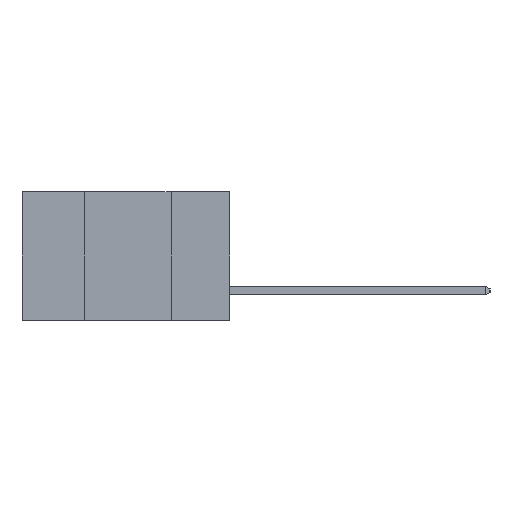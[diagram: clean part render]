
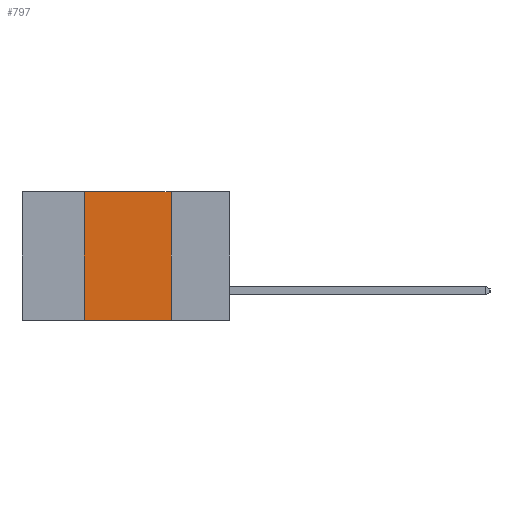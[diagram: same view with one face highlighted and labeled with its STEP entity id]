
A CAD part, left-side view. The second image highlights one B-rep face of the part: STEP entity #797.
In plain terms, the highlighted planar face has unit normal (-1, 0, 0).
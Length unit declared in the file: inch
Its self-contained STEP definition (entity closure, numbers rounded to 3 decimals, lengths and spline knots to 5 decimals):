
#316 = DIRECTION ( 'NONE',  ( 0., -1., 0. ) ) ;
#605 = DIRECTION ( 'NONE',  ( 0., 0., -1. ) ) ;
#797 = ADVANCED_FACE ( 'NONE', ( #4224 ), #5709, .F. ) ;
#1355 = DIRECTION ( 'NONE',  ( 0., 0., -1. ) ) ;
#2136 = DIRECTION ( 'NONE',  ( 1., 0., 0. ) ) ;
#2278 = CARTESIAN_POINT ( 'NONE',  ( 0., 0.17, 0. ) ) ;
#2495 = VERTEX_POINT ( 'NONE', #7505 ) ;
#2647 = AXIS2_PLACEMENT_3D ( 'NONE', #14229, #2136, #1355 ) ;
#2806 = EDGE_CURVE ( 'NONE', #2495, #14706, #14715, .T. ) ;
#3045 = VECTOR ( 'NONE', #605, 39.37008 ) ;
#4089 = ORIENTED_EDGE ( 'NONE', *, *, #2806, .F. ) ;
#4102 = CARTESIAN_POINT ( 'NONE',  ( 0., 0.17, -0.37 ) ) ;
#4224 = FACE_OUTER_BOUND ( 'NONE', #4238, .T. ) ;
#4238 = EDGE_LOOP ( 'NONE', ( #6696, #4089, #9150, #4244 ) ) ;
#4244 = ORIENTED_EDGE ( 'NONE', *, *, #5163, .T. ) ;
#4449 = CARTESIAN_POINT ( 'NONE',  ( 0., 0.42, -0.37 ) ) ;
#4867 = CARTESIAN_POINT ( 'NONE',  ( 0., 0.42, 0. ) ) ;
#5163 = EDGE_CURVE ( 'NONE', #10634, #12291, #5690, .T. ) ;
#5690 = LINE ( 'NONE', #10066, #6448 ) ;
#5709 = PLANE ( 'NONE',  #2647 ) ;
#6445 = DIRECTION ( 'NONE',  ( 0., -1., 0. ) ) ;
#6448 = VECTOR ( 'NONE', #6445, 39.37008 ) ;
#6559 = CARTESIAN_POINT ( 'NONE',  ( 0., 0.17, 0. ) ) ;
#6696 = ORIENTED_EDGE ( 'NONE', *, *, #11804, .F. ) ;
#7505 = CARTESIAN_POINT ( 'NONE',  ( 0., 0.42, 0. ) ) ;
#9150 = ORIENTED_EDGE ( 'NONE', *, *, #12096, .F. ) ;
#10066 = CARTESIAN_POINT ( 'NONE',  ( 0., 0.6, -0.37 ) ) ;
#10634 = VERTEX_POINT ( 'NONE', #4449 ) ;
#10825 = DIRECTION ( 'NONE',  ( 0., 0., 1. ) ) ;
#11586 = VECTOR ( 'NONE', #316, 39.37008 ) ;
#11804 = EDGE_CURVE ( 'NONE', #14706, #12291, #12485, .T. ) ;
#12096 = EDGE_CURVE ( 'NONE', #10634, #2495, #14315, .T. ) ;
#12291 = VERTEX_POINT ( 'NONE', #4102 ) ;
#12445 = CARTESIAN_POINT ( 'NONE',  ( 0., 0.6, 0. ) ) ;
#12485 = LINE ( 'NONE', #6559, #3045 ) ;
#14229 = CARTESIAN_POINT ( 'NONE',  ( 0., 0.6, 0. ) ) ;
#14315 = LINE ( 'NONE', #4867, #14699 ) ;
#14699 = VECTOR ( 'NONE', #10825, 39.37008 ) ;
#14706 = VERTEX_POINT ( 'NONE', #2278 ) ;
#14715 = LINE ( 'NONE', #12445, #11586 ) ;
